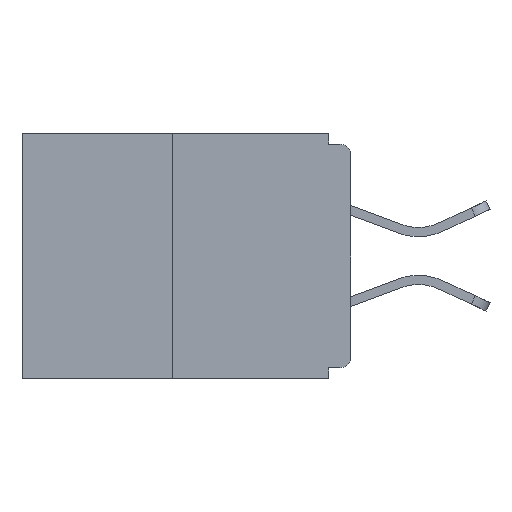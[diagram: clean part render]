
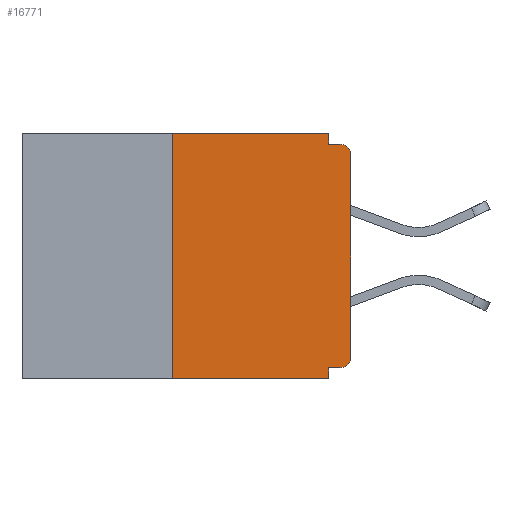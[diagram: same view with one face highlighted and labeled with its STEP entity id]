
A CAD part, left-side view. The second image highlights one B-rep face of the part: STEP entity #16771.
In plain terms, the highlighted planar face has unit normal (-1, 0, 0).
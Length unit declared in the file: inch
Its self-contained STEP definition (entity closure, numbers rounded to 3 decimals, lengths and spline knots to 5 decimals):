
#150 = DIRECTION ( 'NONE',  ( -1., 0., 0. ) ) ;
#640 = VECTOR ( 'NONE', #20532, 39.37008 ) ;
#1382 = CARTESIAN_POINT ( 'NONE',  ( 0., 0.015, -0.015 ) ) ;
#1671 = CIRCLE ( 'NONE', #13479, 0.015 ) ;
#1768 = VECTOR ( 'NONE', #24557, 39.37008 ) ;
#1922 = DIRECTION ( 'NONE',  ( 0., 0., -1. ) ) ;
#2832 = LINE ( 'NONE', #15323, #22763 ) ;
#2912 = DIRECTION ( 'NONE',  ( 0., 0., 1. ) ) ;
#2922 = DIRECTION ( 'NONE',  ( 0., 0., -1. ) ) ;
#3063 = ORIENTED_EDGE ( 'NONE', *, *, #19233, .T. ) ;
#3113 = ORIENTED_EDGE ( 'NONE', *, *, #22598, .F. ) ;
#3143 = ORIENTED_EDGE ( 'NONE', *, *, #19248, .T. ) ;
#3252 = ORIENTED_EDGE ( 'NONE', *, *, #5812, .F. ) ;
#5260 = VECTOR ( 'NONE', #24942, 39.37008 ) ;
#5600 = CARTESIAN_POINT ( 'NONE',  ( 0., 0.031, 0. ) ) ;
#5812 = EDGE_CURVE ( 'NONE', #18288, #15937, #13225, .T. ) ;
#5825 = DIRECTION ( 'NONE',  ( 0., 0., 1. ) ) ;
#5954 = LINE ( 'NONE', #11014, #20787 ) ;
#6096 = CARTESIAN_POINT ( 'NONE',  ( 0., 0., -0.03 ) ) ;
#6321 = DIRECTION ( 'NONE',  ( 1., 0., 0. ) ) ;
#7291 = ORIENTED_EDGE ( 'NONE', *, *, #10683, .T. ) ;
#7479 = CARTESIAN_POINT ( 'NONE',  ( 0., 0.031, -0.343 ) ) ;
#7591 = LINE ( 'NONE', #8787, #640 ) ;
#7851 = VERTEX_POINT ( 'NONE', #11488 ) ;
#7861 = DIRECTION ( 'NONE',  ( 0., -1., 0. ) ) ;
#8331 = VECTOR ( 'NONE', #7861, 39.37008 ) ;
#8575 = CARTESIAN_POINT ( 'NONE',  ( 0., 0.031, -0.343 ) ) ;
#8787 = CARTESIAN_POINT ( 'NONE',  ( 0., 0., -0.015 ) ) ;
#8957 = CARTESIAN_POINT ( 'NONE',  ( 0., 0.46, -0.343 ) ) ;
#9509 = DIRECTION ( 'NONE',  ( -1., 0., 0. ) ) ;
#9580 = ORIENTED_EDGE ( 'NONE', *, *, #11516, .F. ) ;
#10224 = VERTEX_POINT ( 'NONE', #17257 ) ;
#10683 = EDGE_CURVE ( 'NONE', #7851, #21022, #5954, .T. ) ;
#11014 = CARTESIAN_POINT ( 'NONE',  ( 0., 0., 0. ) ) ;
#11149 = CARTESIAN_POINT ( 'NONE',  ( 0., 0.031, -0.328 ) ) ;
#11247 = CARTESIAN_POINT ( 'NONE',  ( 0., 0.46, 0. ) ) ;
#11488 = CARTESIAN_POINT ( 'NONE',  ( 0., 0., -0.313 ) ) ;
#11516 = EDGE_CURVE ( 'NONE', #13891, #10224, #21336, .T. ) ;
#11718 = CARTESIAN_POINT ( 'NONE',  ( 0., 0.015, -0.03 ) ) ;
#11999 = EDGE_LOOP ( 'NONE', ( #21324, #3252, #16061, #17381, #3113, #3143, #7291, #3063, #16949, #9580 ) ) ;
#12216 = VECTOR ( 'NONE', #2922, 39.37008 ) ;
#12461 = AXIS2_PLACEMENT_3D ( 'NONE', #17921, #6321, #23739 ) ;
#12478 = VERTEX_POINT ( 'NONE', #11149 ) ;
#13211 = DIRECTION ( 'NONE',  ( 0., 1., 0. ) ) ;
#13225 = LINE ( 'NONE', #17431, #17498 ) ;
#13479 = AXIS2_PLACEMENT_3D ( 'NONE', #13644, #9509, #21423 ) ;
#13644 = CARTESIAN_POINT ( 'NONE',  ( 0., 0.015, -0.313 ) ) ;
#13891 = VERTEX_POINT ( 'NONE', #21030 ) ;
#14278 = AXIS2_PLACEMENT_3D ( 'NONE', #11718, #150, #1922 ) ;
#14380 = LINE ( 'NONE', #11247, #8331 ) ;
#14860 = EDGE_CURVE ( 'NONE', #10224, #22474, #7591, .T. ) ;
#15323 = CARTESIAN_POINT ( 'NONE',  ( 0., 0., -0.328 ) ) ;
#15850 = CIRCLE ( 'NONE', #14278, 0.015 ) ;
#15937 = VERTEX_POINT ( 'NONE', #23967 ) ;
#15998 = PLANE ( 'NONE',  #12461 ) ;
#16061 = ORIENTED_EDGE ( 'NONE', *, *, #16406, .T. ) ;
#16406 = EDGE_CURVE ( 'NONE', #18288, #22129, #16871, .T. ) ;
#16771 = ADVANCED_FACE ( 'NONE', ( #19279 ), #15998, .F. ) ;
#16871 = LINE ( 'NONE', #8957, #1768 ) ;
#16949 = ORIENTED_EDGE ( 'NONE', *, *, #14860, .F. ) ;
#17257 = CARTESIAN_POINT ( 'NONE',  ( 0., 0.031, -0.015 ) ) ;
#17381 = ORIENTED_EDGE ( 'NONE', *, *, #22342, .F. ) ;
#17431 = CARTESIAN_POINT ( 'NONE',  ( 0., 0.25, 0. ) ) ;
#17498 = VECTOR ( 'NONE', #5825, 39.37008 ) ;
#17893 = CARTESIAN_POINT ( 'NONE',  ( 0., 0.015, -0.328 ) ) ;
#17921 = CARTESIAN_POINT ( 'NONE',  ( 0., 0.46, 0. ) ) ;
#18288 = VERTEX_POINT ( 'NONE', #21713 ) ;
#19233 = EDGE_CURVE ( 'NONE', #21022, #22474, #15850, .T. ) ;
#19248 = EDGE_CURVE ( 'NONE', #19879, #7851, #1671, .T. ) ;
#19279 = FACE_OUTER_BOUND ( 'NONE', #11999, .T. ) ;
#19879 = VERTEX_POINT ( 'NONE', #17893 ) ;
#20532 = DIRECTION ( 'NONE',  ( 0., -1., 0. ) ) ;
#20787 = VECTOR ( 'NONE', #2912, 39.37008 ) ;
#21022 = VERTEX_POINT ( 'NONE', #6096 ) ;
#21030 = CARTESIAN_POINT ( 'NONE',  ( 0., 0.031, 0. ) ) ;
#21324 = ORIENTED_EDGE ( 'NONE', *, *, #21456, .F. ) ;
#21336 = LINE ( 'NONE', #5600, #5260 ) ;
#21423 = DIRECTION ( 'NONE',  ( 0., 0., -1. ) ) ;
#21456 = EDGE_CURVE ( 'NONE', #15937, #13891, #14380, .T. ) ;
#21713 = CARTESIAN_POINT ( 'NONE',  ( 0., 0.25, -0.343 ) ) ;
#22129 = VERTEX_POINT ( 'NONE', #7479 ) ;
#22342 = EDGE_CURVE ( 'NONE', #12478, #22129, #22442, .T. ) ;
#22442 = LINE ( 'NONE', #8575, #12216 ) ;
#22474 = VERTEX_POINT ( 'NONE', #1382 ) ;
#22598 = EDGE_CURVE ( 'NONE', #19879, #12478, #2832, .T. ) ;
#22763 = VECTOR ( 'NONE', #13211, 39.37008 ) ;
#23739 = DIRECTION ( 'NONE',  ( 0., 0., -1. ) ) ;
#23967 = CARTESIAN_POINT ( 'NONE',  ( 0., 0.25, 0. ) ) ;
#24557 = DIRECTION ( 'NONE',  ( 0., -1., 0. ) ) ;
#24942 = DIRECTION ( 'NONE',  ( 0., 0., -1. ) ) ;
